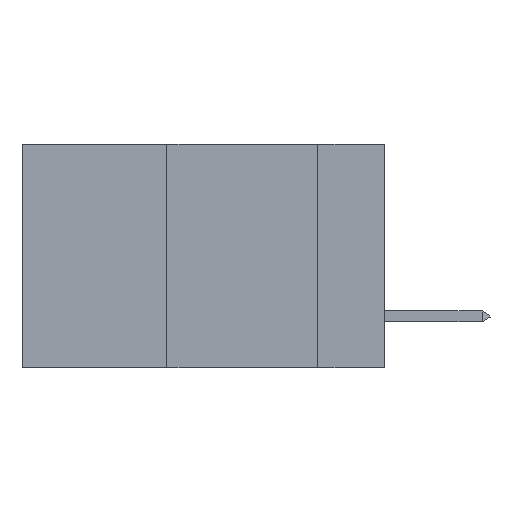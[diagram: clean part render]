
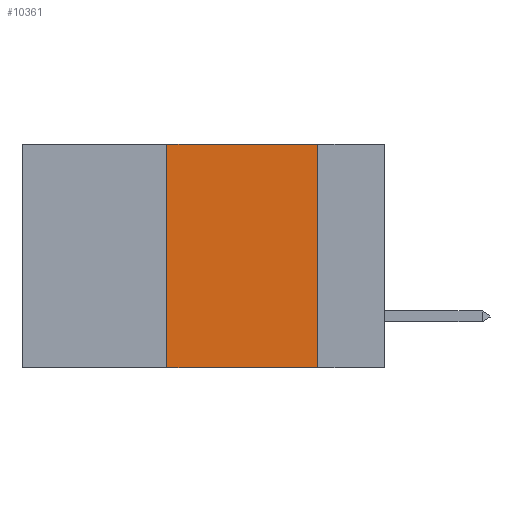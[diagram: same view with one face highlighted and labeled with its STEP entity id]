
A CAD part, left-side view. The second image highlights one B-rep face of the part: STEP entity #10361.
In plain terms, the highlighted planar face has unit normal (-1, 0, 0).
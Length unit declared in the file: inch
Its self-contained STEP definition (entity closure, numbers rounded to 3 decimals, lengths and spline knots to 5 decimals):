
#164 = CARTESIAN_POINT ( 'NONE',  ( 0., 0.11, 0. ) ) ;
#314 = CARTESIAN_POINT ( 'NONE',  ( 0., 0.36, 0. ) ) ;
#612 = DIRECTION ( 'NONE',  ( 0., 0., -1. ) ) ;
#817 = VERTEX_POINT ( 'NONE', #16466 ) ;
#1018 = CARTESIAN_POINT ( 'NONE',  ( 0., 0.6, 0. ) ) ;
#1990 = PLANE ( 'NONE',  #8119 ) ;
#2481 = CARTESIAN_POINT ( 'NONE',  ( 0., 0.36, 0. ) ) ;
#2801 = ORIENTED_EDGE ( 'NONE', *, *, #5848, .F. ) ;
#5559 = DIRECTION ( 'NONE',  ( 0., -1., 0. ) ) ;
#5848 = EDGE_CURVE ( 'NONE', #9100, #8141, #18294, .T. ) ;
#6267 = DIRECTION ( 'NONE',  ( 0., 0., -1. ) ) ;
#6616 = FACE_OUTER_BOUND ( 'NONE', #19269, .T. ) ;
#7465 = EDGE_CURVE ( 'NONE', #817, #9379, #18969, .T. ) ;
#7549 = ORIENTED_EDGE ( 'NONE', *, *, #12300, .F. ) ;
#8119 = AXIS2_PLACEMENT_3D ( 'NONE', #10784, #10906, #6267 ) ;
#8141 = VERTEX_POINT ( 'NONE', #164 ) ;
#8383 = VECTOR ( 'NONE', #5559, 39.37008 ) ;
#9100 = VERTEX_POINT ( 'NONE', #314 ) ;
#9379 = VERTEX_POINT ( 'NONE', #14736 ) ;
#9614 = CARTESIAN_POINT ( 'NONE',  ( 0., 0.11, 0. ) ) ;
#10361 = ADVANCED_FACE ( 'NONE', ( #6616 ), #1990, .F. ) ;
#10784 = CARTESIAN_POINT ( 'NONE',  ( 0., 0.6, 0. ) ) ;
#10793 = VECTOR ( 'NONE', #15951, 39.37008 ) ;
#10906 = DIRECTION ( 'NONE',  ( 1., 0., 0. ) ) ;
#11697 = DIRECTION ( 'NONE',  ( 0., 0., 1. ) ) ;
#12299 = VECTOR ( 'NONE', #612, 39.37008 ) ;
#12300 = EDGE_CURVE ( 'NONE', #8141, #9379, #15134, .T. ) ;
#13710 = ORIENTED_EDGE ( 'NONE', *, *, #7465, .T. ) ;
#14022 = ORIENTED_EDGE ( 'NONE', *, *, #19330, .F. ) ;
#14345 = CARTESIAN_POINT ( 'NONE',  ( 0., 0.6, -0.37 ) ) ;
#14354 = VECTOR ( 'NONE', #11697, 39.37008 ) ;
#14736 = CARTESIAN_POINT ( 'NONE',  ( 0., 0.11, -0.37 ) ) ;
#15134 = LINE ( 'NONE', #9614, #12299 ) ;
#15310 = LINE ( 'NONE', #2481, #14354 ) ;
#15951 = DIRECTION ( 'NONE',  ( 0., -1., 0. ) ) ;
#16466 = CARTESIAN_POINT ( 'NONE',  ( 0., 0.36, -0.37 ) ) ;
#18294 = LINE ( 'NONE', #1018, #10793 ) ;
#18969 = LINE ( 'NONE', #14345, #8383 ) ;
#19269 = EDGE_LOOP ( 'NONE', ( #7549, #2801, #14022, #13710 ) ) ;
#19330 = EDGE_CURVE ( 'NONE', #817, #9100, #15310, .T. ) ;
